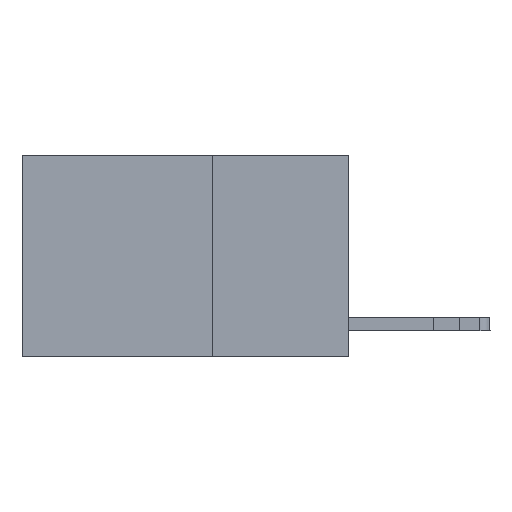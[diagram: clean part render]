
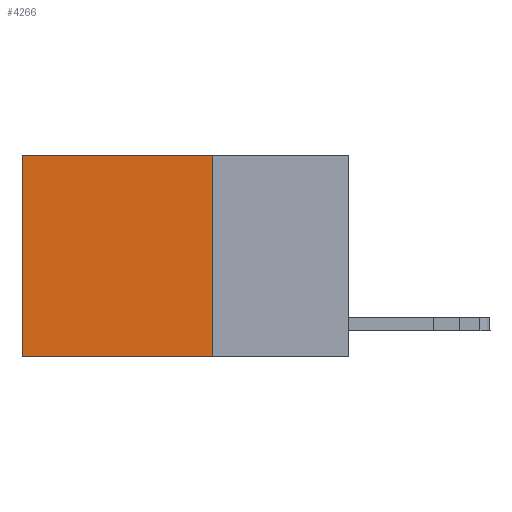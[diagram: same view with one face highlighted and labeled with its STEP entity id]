
A CAD part, left-side view. The second image highlights one B-rep face of the part: STEP entity #4266.
In plain terms, the highlighted planar face has unit normal (-1, 0, 0).
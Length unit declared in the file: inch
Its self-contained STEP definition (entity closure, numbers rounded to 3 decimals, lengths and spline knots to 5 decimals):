
#7 = ORIENTED_EDGE ( 'NONE', *, *, #2924, .T. ) ;
#363 = CARTESIAN_POINT ( 'NONE',  ( 0.2625, 0.25, 0. ) ) ;
#396 = LINE ( 'NONE', #11167, #10392 ) ;
#756 = DIRECTION ( 'NONE',  ( 0., 0., -1. ) ) ;
#1312 = VECTOR ( 'NONE', #756, 39.37008 ) ;
#1361 = VERTEX_POINT ( 'NONE', #8078 ) ;
#1651 = AXIS2_PLACEMENT_3D ( 'NONE', #12258, #2457, #3524 ) ;
#1728 = LINE ( 'NONE', #5600, #1312 ) ;
#1792 = VERTEX_POINT ( 'NONE', #363 ) ;
#2048 = DIRECTION ( 'NONE',  ( 0., 1., 0. ) ) ;
#2126 = VECTOR ( 'NONE', #4515, 39.37008 ) ;
#2177 = CARTESIAN_POINT ( 'NONE',  ( 0.2625, 0.25, -0.37 ) ) ;
#2457 = DIRECTION ( 'NONE',  ( 1., 0., 0. ) ) ;
#2924 = EDGE_CURVE ( 'NONE', #1792, #7559, #396, .T. ) ;
#3524 = DIRECTION ( 'NONE',  ( 0., 0., -1. ) ) ;
#4266 = ADVANCED_FACE ( 'NONE', ( #7304 ), #11170, .F. ) ;
#4425 = DIRECTION ( 'NONE',  ( 0., 1., 0. ) ) ;
#4515 = DIRECTION ( 'NONE',  ( 0., 0., -1. ) ) ;
#5447 = CARTESIAN_POINT ( 'NONE',  ( 0.2625, 0.6, 0. ) ) ;
#5600 = CARTESIAN_POINT ( 'NONE',  ( 0.2625, 0.25, 0. ) ) ;
#6998 = EDGE_CURVE ( 'NONE', #7559, #11399, #7578, .T. ) ;
#7021 = LINE ( 'NONE', #2177, #11139 ) ;
#7304 = FACE_OUTER_BOUND ( 'NONE', #9434, .T. ) ;
#7559 = VERTEX_POINT ( 'NONE', #8955 ) ;
#7578 = LINE ( 'NONE', #5447, #2126 ) ;
#8078 = CARTESIAN_POINT ( 'NONE',  ( 0.2625, 0.25, -0.37 ) ) ;
#8384 = EDGE_CURVE ( 'NONE', #1792, #1361, #1728, .T. ) ;
#8698 = ORIENTED_EDGE ( 'NONE', *, *, #6998, .T. ) ;
#8955 = CARTESIAN_POINT ( 'NONE',  ( 0.2625, 0.6, 0. ) ) ;
#9058 = EDGE_CURVE ( 'NONE', #1361, #11399, #7021, .T. ) ;
#9221 = ORIENTED_EDGE ( 'NONE', *, *, #9058, .F. ) ;
#9332 = ORIENTED_EDGE ( 'NONE', *, *, #8384, .F. ) ;
#9434 = EDGE_LOOP ( 'NONE', ( #8698, #9221, #9332, #7 ) ) ;
#10392 = VECTOR ( 'NONE', #4425, 39.37008 ) ;
#11139 = VECTOR ( 'NONE', #2048, 39.37008 ) ;
#11167 = CARTESIAN_POINT ( 'NONE',  ( 0.2625, 0.25, 0. ) ) ;
#11170 = PLANE ( 'NONE',  #1651 ) ;
#11176 = CARTESIAN_POINT ( 'NONE',  ( 0.2625, 0.6, -0.37 ) ) ;
#11399 = VERTEX_POINT ( 'NONE', #11176 ) ;
#12258 = CARTESIAN_POINT ( 'NONE',  ( 0.2625, 0.25, 0. ) ) ;
